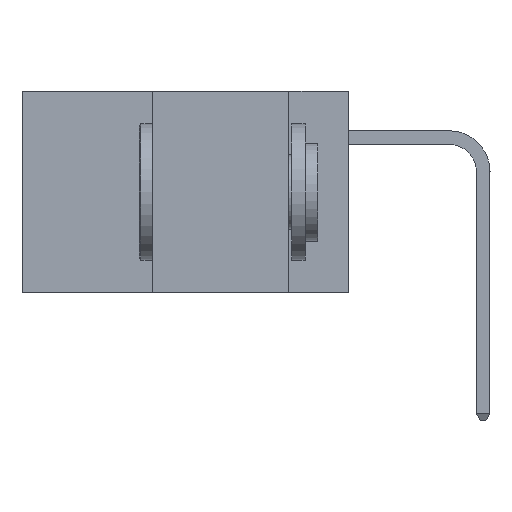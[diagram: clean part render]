
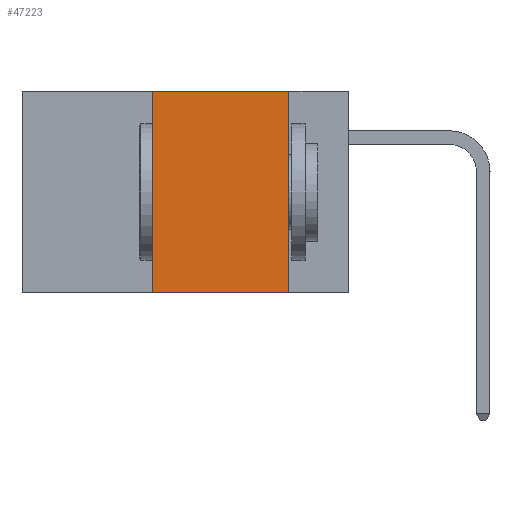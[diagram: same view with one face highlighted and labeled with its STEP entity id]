
A CAD part, left-side view. The second image highlights one B-rep face of the part: STEP entity #47223.
In plain terms, the highlighted planar face has unit normal (-1, 0, 0).
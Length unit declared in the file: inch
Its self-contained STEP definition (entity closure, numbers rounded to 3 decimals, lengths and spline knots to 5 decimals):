
#492 = FACE_OUTER_BOUND ( 'NONE', #28159, .T. ) ;
#7171 = DIRECTION ( 'NONE',  ( 1., 0., 0. ) ) ;
#7270 = EDGE_CURVE ( 'NONE', #37433, #30029, #19148, .T. ) ;
#7310 = LINE ( 'NONE', #32522, #18189 ) ;
#10145 = DIRECTION ( 'NONE',  ( 0., 0., -1. ) ) ;
#10526 = EDGE_CURVE ( 'NONE', #37433, #44967, #28214, .T. ) ;
#11799 = VERTEX_POINT ( 'NONE', #29009 ) ;
#12359 = AXIS2_PLACEMENT_3D ( 'NONE', #43733, #7171, #21557 ) ;
#13519 = CARTESIAN_POINT ( 'NONE',  ( 0., 0.11, -0.37 ) ) ;
#13904 = ORIENTED_EDGE ( 'NONE', *, *, #7270, .T. ) ;
#14708 = DIRECTION ( 'NONE',  ( 0., -1., 0. ) ) ;
#16759 = ORIENTED_EDGE ( 'NONE', *, *, #30899, .F. ) ;
#18189 = VECTOR ( 'NONE', #10145, 39.37008 ) ;
#18949 = CARTESIAN_POINT ( 'NONE',  ( 0., 0.36, -0.37 ) ) ;
#19148 = LINE ( 'NONE', #38307, #43117 ) ;
#19736 = DIRECTION ( 'NONE',  ( 0., 0., 1. ) ) ;
#19890 = CARTESIAN_POINT ( 'NONE',  ( 0., 0.36, 0. ) ) ;
#21012 = VECTOR ( 'NONE', #14708, 39.37008 ) ;
#21557 = DIRECTION ( 'NONE',  ( 0., 0., -1. ) ) ;
#25187 = ORIENTED_EDGE ( 'NONE', *, *, #30218, .F. ) ;
#26926 = DIRECTION ( 'NONE',  ( 0., -1., 0. ) ) ;
#28159 = EDGE_LOOP ( 'NONE', ( #25187, #16759, #34046, #13904 ) ) ;
#28214 = LINE ( 'NONE', #19890, #43664 ) ;
#29009 = CARTESIAN_POINT ( 'NONE',  ( 0., 0.11, 0. ) ) ;
#30029 = VERTEX_POINT ( 'NONE', #13519 ) ;
#30218 = EDGE_CURVE ( 'NONE', #11799, #30029, #7310, .T. ) ;
#30899 = EDGE_CURVE ( 'NONE', #44967, #11799, #34149, .T. ) ;
#32522 = CARTESIAN_POINT ( 'NONE',  ( 0., 0.11, 0. ) ) ;
#34046 = ORIENTED_EDGE ( 'NONE', *, *, #10526, .F. ) ;
#34149 = LINE ( 'NONE', #44251, #21012 ) ;
#35477 = CARTESIAN_POINT ( 'NONE',  ( 0., 0.36, 0. ) ) ;
#37433 = VERTEX_POINT ( 'NONE', #18949 ) ;
#38307 = CARTESIAN_POINT ( 'NONE',  ( 0., 0.6, -0.37 ) ) ;
#40382 = PLANE ( 'NONE',  #12359 ) ;
#43117 = VECTOR ( 'NONE', #26926, 39.37008 ) ;
#43664 = VECTOR ( 'NONE', #19736, 39.37008 ) ;
#43733 = CARTESIAN_POINT ( 'NONE',  ( 0., 0.6, 0. ) ) ;
#44251 = CARTESIAN_POINT ( 'NONE',  ( 0., 0.6, 0. ) ) ;
#44967 = VERTEX_POINT ( 'NONE', #35477 ) ;
#47223 = ADVANCED_FACE ( 'NONE', ( #492 ), #40382, .F. ) ;
